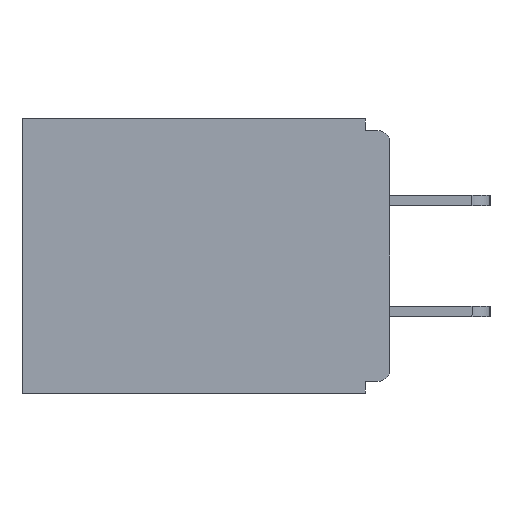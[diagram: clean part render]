
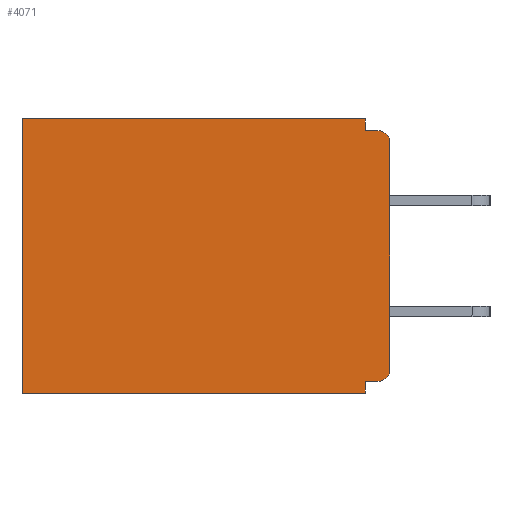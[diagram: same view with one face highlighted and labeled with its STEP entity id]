
A CAD part, left-side view. The second image highlights one B-rep face of the part: STEP entity #4071.
In plain terms, the highlighted planar face has unit normal (-1, 0, 0).
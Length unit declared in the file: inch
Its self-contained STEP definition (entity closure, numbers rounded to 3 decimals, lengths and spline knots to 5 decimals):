
#19 = CARTESIAN_POINT ( 'NONE',  ( 0.298, 0.015, -0.328 ) ) ;
#204 = LINE ( 'NONE', #1423, #2517 ) ;
#477 = DIRECTION ( 'NONE',  ( 0., 0., -1. ) ) ;
#779 = ORIENTED_EDGE ( 'NONE', *, *, #8711, .T. ) ;
#839 = DIRECTION ( 'NONE',  ( 0., 0., -1. ) ) ;
#908 = VERTEX_POINT ( 'NONE', #5102 ) ;
#1010 = DIRECTION ( 'NONE',  ( 1., 0., 0. ) ) ;
#1035 = DIRECTION ( 'NONE',  ( 0., 0., -1. ) ) ;
#1166 = VECTOR ( 'NONE', #8464, 39.37008 ) ;
#1197 = LINE ( 'NONE', #10474, #5489 ) ;
#1358 = ORIENTED_EDGE ( 'NONE', *, *, #6070, .T. ) ;
#1423 = CARTESIAN_POINT ( 'NONE',  ( 0.298, 0., -0.343 ) ) ;
#1500 = VERTEX_POINT ( 'NONE', #3551 ) ;
#1685 = VERTEX_POINT ( 'NONE', #19 ) ;
#1863 = CIRCLE ( 'NONE', #9298, 0.015 ) ;
#1874 = ORIENTED_EDGE ( 'NONE', *, *, #7761, .F. ) ;
#1892 = VERTEX_POINT ( 'NONE', #7326 ) ;
#2164 = CARTESIAN_POINT ( 'NONE',  ( 0.298, 0., -0.015 ) ) ;
#2289 = ORIENTED_EDGE ( 'NONE', *, *, #9170, .F. ) ;
#2409 = CARTESIAN_POINT ( 'NONE',  ( 0.298, 0., 0. ) ) ;
#2517 = VECTOR ( 'NONE', #7611, 39.37008 ) ;
#2751 = EDGE_CURVE ( 'NONE', #4374, #10021, #7355, .T. ) ;
#2900 = EDGE_CURVE ( 'NONE', #8153, #908, #3377, .T. ) ;
#2922 = EDGE_LOOP ( 'NONE', ( #4310, #9443, #2289, #1358, #10546, #1874, #3118, #3290, #779, #4084 ) ) ;
#3118 = ORIENTED_EDGE ( 'NONE', *, *, #5951, .F. ) ;
#3170 = EDGE_CURVE ( 'NONE', #4637, #1500, #8140, .T. ) ;
#3290 = ORIENTED_EDGE ( 'NONE', *, *, #4673, .F. ) ;
#3377 = LINE ( 'NONE', #6342, #6497 ) ;
#3551 = CARTESIAN_POINT ( 'NONE',  ( 0.298, 0.015, -0.015 ) ) ;
#3578 = CIRCLE ( 'NONE', #4034, 0.015 ) ;
#3683 = CARTESIAN_POINT ( 'NONE',  ( 0.298, 0.015, -0.313 ) ) ;
#4034 = AXIS2_PLACEMENT_3D ( 'NONE', #3683, #8940, #9911 ) ;
#4071 = ADVANCED_FACE ( 'NONE', ( #8514 ), #7149, .F. ) ;
#4084 = ORIENTED_EDGE ( 'NONE', *, *, #2751, .F. ) ;
#4310 = ORIENTED_EDGE ( 'NONE', *, *, #5219, .T. ) ;
#4374 = VERTEX_POINT ( 'NONE', #11380 ) ;
#4448 = DIRECTION ( 'NONE',  ( 0., 0., -1. ) ) ;
#4637 = VERTEX_POINT ( 'NONE', #5049 ) ;
#4673 = EDGE_CURVE ( 'NONE', #1685, #1892, #1197, .T. ) ;
#4731 = LINE ( 'NONE', #2409, #10293 ) ;
#4901 = DIRECTION ( 'NONE',  ( 0., -1., 0. ) ) ;
#5049 = CARTESIAN_POINT ( 'NONE',  ( 0.298, 0.031, -0.015 ) ) ;
#5102 = CARTESIAN_POINT ( 'NONE',  ( 0.298, 0.46, -0.343 ) ) ;
#5219 = EDGE_CURVE ( 'NONE', #4374, #1500, #1863, .T. ) ;
#5270 = VECTOR ( 'NONE', #477, 39.37008 ) ;
#5435 = CARTESIAN_POINT ( 'NONE',  ( 0.298, 0.031, -0.343 ) ) ;
#5452 = CARTESIAN_POINT ( 'NONE',  ( 0.298, 0.031, 0. ) ) ;
#5489 = VECTOR ( 'NONE', #6982, 39.37008 ) ;
#5578 = CARTESIAN_POINT ( 'NONE',  ( 0.298, 0.031, -0.343 ) ) ;
#5834 = AXIS2_PLACEMENT_3D ( 'NONE', #9791, #1010, #4448 ) ;
#5951 = EDGE_CURVE ( 'NONE', #1892, #7546, #7137, .T. ) ;
#6047 = DIRECTION ( 'NONE',  ( 0., 1., 0. ) ) ;
#6070 = EDGE_CURVE ( 'NONE', #6380, #8153, #4731, .T. ) ;
#6142 = CARTESIAN_POINT ( 'NONE',  ( 0.298, 0., 0. ) ) ;
#6224 = VECTOR ( 'NONE', #839, 39.37008 ) ;
#6342 = CARTESIAN_POINT ( 'NONE',  ( 0.298, 0.46, 0. ) ) ;
#6380 = VERTEX_POINT ( 'NONE', #5452 ) ;
#6497 = VECTOR ( 'NONE', #7085, 39.37008 ) ;
#6982 = DIRECTION ( 'NONE',  ( 0., 1., 0. ) ) ;
#7085 = DIRECTION ( 'NONE',  ( 0., 0., -1. ) ) ;
#7137 = LINE ( 'NONE', #5435, #1166 ) ;
#7149 = PLANE ( 'NONE',  #5834 ) ;
#7157 = CARTESIAN_POINT ( 'NONE',  ( 0.298, 0.031, -0.343 ) ) ;
#7326 = CARTESIAN_POINT ( 'NONE',  ( 0.298, 0.031, -0.328 ) ) ;
#7355 = LINE ( 'NONE', #6142, #6224 ) ;
#7546 = VERTEX_POINT ( 'NONE', #7157 ) ;
#7600 = VECTOR ( 'NONE', #4901, 39.37008 ) ;
#7611 = DIRECTION ( 'NONE',  ( 0., 1., 0. ) ) ;
#7761 = EDGE_CURVE ( 'NONE', #7546, #908, #204, .T. ) ;
#7998 = CARTESIAN_POINT ( 'NONE',  ( 0.298, 0.015, -0.03 ) ) ;
#8140 = LINE ( 'NONE', #2164, #7600 ) ;
#8153 = VERTEX_POINT ( 'NONE', #8275 ) ;
#8275 = CARTESIAN_POINT ( 'NONE',  ( 0.298, 0.46, 0. ) ) ;
#8464 = DIRECTION ( 'NONE',  ( 0., 0., -1. ) ) ;
#8514 = FACE_OUTER_BOUND ( 'NONE', #2922, .T. ) ;
#8607 = DIRECTION ( 'NONE',  ( -1., 0., 0. ) ) ;
#8659 = CARTESIAN_POINT ( 'NONE',  ( 0.298, 0., -0.313 ) ) ;
#8711 = EDGE_CURVE ( 'NONE', #1685, #10021, #3578, .T. ) ;
#8940 = DIRECTION ( 'NONE',  ( -1., 0., 0. ) ) ;
#9170 = EDGE_CURVE ( 'NONE', #6380, #4637, #9994, .T. ) ;
#9298 = AXIS2_PLACEMENT_3D ( 'NONE', #7998, #8607, #1035 ) ;
#9443 = ORIENTED_EDGE ( 'NONE', *, *, #3170, .F. ) ;
#9791 = CARTESIAN_POINT ( 'NONE',  ( 0.298, 0., 0. ) ) ;
#9911 = DIRECTION ( 'NONE',  ( 0., 0., -1. ) ) ;
#9994 = LINE ( 'NONE', #5578, #5270 ) ;
#10021 = VERTEX_POINT ( 'NONE', #8659 ) ;
#10293 = VECTOR ( 'NONE', #6047, 39.37008 ) ;
#10474 = CARTESIAN_POINT ( 'NONE',  ( 0.298, 0., -0.328 ) ) ;
#10546 = ORIENTED_EDGE ( 'NONE', *, *, #2900, .T. ) ;
#11380 = CARTESIAN_POINT ( 'NONE',  ( 0.298, 0., -0.03 ) ) ;
